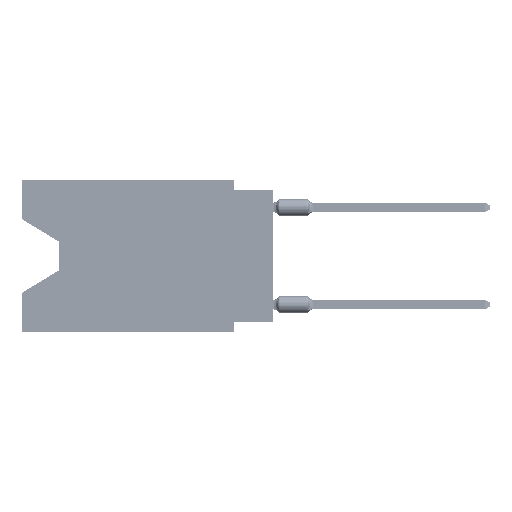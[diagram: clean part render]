
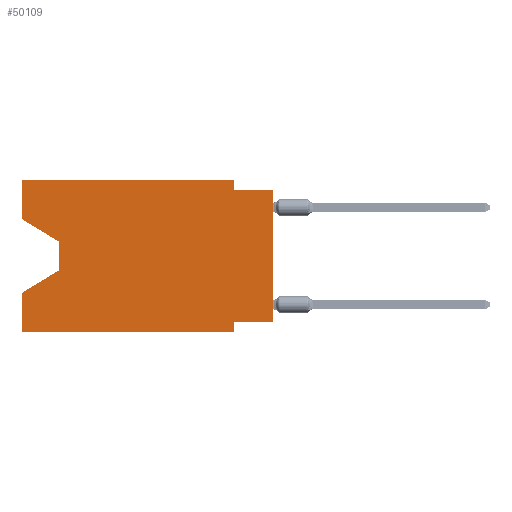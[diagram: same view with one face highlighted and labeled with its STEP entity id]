
A CAD part, left-side view. The second image highlights one B-rep face of the part: STEP entity #50109.
In plain terms, the highlighted planar face has unit normal (-1, 0, 0).
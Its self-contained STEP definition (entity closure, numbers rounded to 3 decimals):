
#294 = VECTOR ( 'NONE', #69020, 1000. ) ;
#540 = DIRECTION ( 'NONE',  ( 0., -0.855, -0.519 ) ) ;
#623 = VECTOR ( 'NONE', #20585, 1000. ) ;
#2536 = VECTOR ( 'NONE', #59186, 1000. ) ;
#3504 = LINE ( 'NONE', #13956, #27355 ) ;
#3783 = LINE ( 'NONE', #47418, #16172 ) ;
#3912 = CARTESIAN_POINT ( 'NONE',  ( 0., 0., -0.635 ) ) ;
#4102 = CARTESIAN_POINT ( 'NONE',  ( 0., 2.54, -0.635 ) ) ;
#5172 = EDGE_CURVE ( 'NONE', #53596, #12329, #67324, .T. ) ;
#5180 = DIRECTION ( 'NONE',  ( 0., 0., -1. ) ) ;
#5236 = CARTESIAN_POINT ( 'NONE',  ( 0., 2.54, 0. ) ) ;
#5905 = ORIENTED_EDGE ( 'NONE', *, *, #60990, .F. ) ;
#6572 = EDGE_CURVE ( 'NONE', #6758, #55986, #24135, .T. ) ;
#6710 = EDGE_CURVE ( 'NONE', #51719, #12329, #8767, .T. ) ;
#6758 = VERTEX_POINT ( 'NONE', #38417 ) ;
#7532 = VERTEX_POINT ( 'NONE', #47621 ) ;
#7978 = CARTESIAN_POINT ( 'NONE',  ( 0., 13.97, -5.893 ) ) ;
#8767 = LINE ( 'NONE', #68135, #49647 ) ;
#10934 = EDGE_CURVE ( 'NONE', #21162, #53596, #31656, .T. ) ;
#11527 = DIRECTION ( 'NONE',  ( 0., 0., -1. ) ) ;
#12329 = VERTEX_POINT ( 'NONE', #28483 ) ;
#13956 = CARTESIAN_POINT ( 'NONE',  ( 0., 16.383, 0. ) ) ;
#16172 = VECTOR ( 'NONE', #20525, 1000. ) ;
#16595 = CARTESIAN_POINT ( 'NONE',  ( 0., 16.383, -2.546 ) ) ;
#17755 = VERTEX_POINT ( 'NONE', #43179 ) ;
#20525 = DIRECTION ( 'NONE',  ( 0., 0., 1. ) ) ;
#20585 = DIRECTION ( 'NONE',  ( 0., 0.855, -0.519 ) ) ;
#21162 = VERTEX_POINT ( 'NONE', #23049 ) ;
#21661 = CARTESIAN_POINT ( 'NONE',  ( 0., 2.54, 0. ) ) ;
#22603 = CARTESIAN_POINT ( 'NONE',  ( 0., 16.383, 0. ) ) ;
#23049 = CARTESIAN_POINT ( 'NONE',  ( 0., 0., -9.271 ) ) ;
#24135 = LINE ( 'NONE', #61195, #56314 ) ;
#25287 = VECTOR ( 'NONE', #30642, 1000. ) ;
#25675 = ORIENTED_EDGE ( 'NONE', *, *, #6710, .T. ) ;
#25848 = ORIENTED_EDGE ( 'NONE', *, *, #32388, .F. ) ;
#27098 = LINE ( 'NONE', #16595, #43130 ) ;
#27355 = VECTOR ( 'NONE', #46805, 1000. ) ;
#27444 = DIRECTION ( 'NONE',  ( 0., 1., 0. ) ) ;
#27961 = ORIENTED_EDGE ( 'NONE', *, *, #65818, .F. ) ;
#28483 = CARTESIAN_POINT ( 'NONE',  ( 0., 2.54, -9.906 ) ) ;
#29732 = DIRECTION ( 'NONE',  ( 0., -1., 0. ) ) ;
#29880 = AXIS2_PLACEMENT_3D ( 'NONE', #41851, #31728, #5180 ) ;
#30098 = DIRECTION ( 'NONE',  ( 0., -1., 0. ) ) ;
#30329 = ORIENTED_EDGE ( 'NONE', *, *, #45778, .F. ) ;
#30642 = DIRECTION ( 'NONE',  ( 0., 0., -1. ) ) ;
#30957 = LINE ( 'NONE', #48055, #294 ) ;
#31656 = LINE ( 'NONE', #52958, #46522 ) ;
#31728 = DIRECTION ( 'NONE',  ( 1., 0., 0. ) ) ;
#31939 = LINE ( 'NONE', #58147, #2536 ) ;
#32388 = EDGE_CURVE ( 'NONE', #54689, #66324, #38411, .T. ) ;
#34067 = VERTEX_POINT ( 'NONE', #3912 ) ;
#38411 = LINE ( 'NONE', #21661, #49510 ) ;
#38417 = CARTESIAN_POINT ( 'NONE',  ( 0., 13.97, -4.013 ) ) ;
#39183 = DIRECTION ( 'NONE',  ( 0., 0., -1. ) ) ;
#41786 = ORIENTED_EDGE ( 'NONE', *, *, #48623, .T. ) ;
#41851 = CARTESIAN_POINT ( 'NONE',  ( 0., 16.383, 0. ) ) ;
#42254 = CARTESIAN_POINT ( 'NONE',  ( 0., 2.54, -9.271 ) ) ;
#42256 = LINE ( 'NONE', #59036, #623 ) ;
#42548 = FACE_OUTER_BOUND ( 'NONE', #49170, .T. ) ;
#43130 = VECTOR ( 'NONE', #540, 1000. ) ;
#43179 = CARTESIAN_POINT ( 'NONE',  ( 0., 16.383, -7.36 ) ) ;
#43508 = ORIENTED_EDGE ( 'NONE', *, *, #10934, .F. ) ;
#44022 = ORIENTED_EDGE ( 'NONE', *, *, #6572, .T. ) ;
#45778 = EDGE_CURVE ( 'NONE', #65018, #54689, #46466, .T. ) ;
#46466 = LINE ( 'NONE', #47170, #50040 ) ;
#46522 = VECTOR ( 'NONE', #27444, 1000. ) ;
#46805 = DIRECTION ( 'NONE',  ( 0., 0., 1. ) ) ;
#46900 = EDGE_CURVE ( 'NONE', #7532, #65018, #3783, .T. ) ;
#47170 = CARTESIAN_POINT ( 'NONE',  ( 0., 16.383, 0. ) ) ;
#47418 = CARTESIAN_POINT ( 'NONE',  ( 0., 16.383, 0. ) ) ;
#47621 = CARTESIAN_POINT ( 'NONE',  ( 0., 16.383, -2.546 ) ) ;
#48055 = CARTESIAN_POINT ( 'NONE',  ( 0., 0., 0. ) ) ;
#48623 = EDGE_CURVE ( 'NONE', #7532, #6758, #27098, .T. ) ;
#49170 = EDGE_LOOP ( 'NONE', ( #41786, #44022, #50064, #27961, #25675, #57112, #43508, #57638, #5905, #25848, #30329, #62184 ) ) ;
#49510 = VECTOR ( 'NONE', #11527, 1000. ) ;
#49647 = VECTOR ( 'NONE', #30098, 1000. ) ;
#50040 = VECTOR ( 'NONE', #29732, 1000. ) ;
#50064 = ORIENTED_EDGE ( 'NONE', *, *, #66075, .T. ) ;
#50109 = ADVANCED_FACE ( 'NONE', ( #42548 ), #57940, .F. ) ;
#51719 = VERTEX_POINT ( 'NONE', #51935 ) ;
#51935 = CARTESIAN_POINT ( 'NONE',  ( 0., 16.383, -9.906 ) ) ;
#51950 = CARTESIAN_POINT ( 'NONE',  ( 0., 2.54, -9.906 ) ) ;
#52958 = CARTESIAN_POINT ( 'NONE',  ( 0., 0., -9.271 ) ) ;
#53596 = VERTEX_POINT ( 'NONE', #42254 ) ;
#54689 = VERTEX_POINT ( 'NONE', #5236 ) ;
#55986 = VERTEX_POINT ( 'NONE', #7978 ) ;
#56314 = VECTOR ( 'NONE', #39183, 1000. ) ;
#57112 = ORIENTED_EDGE ( 'NONE', *, *, #5172, .F. ) ;
#57638 = ORIENTED_EDGE ( 'NONE', *, *, #62612, .T. ) ;
#57940 = PLANE ( 'NONE',  #29880 ) ;
#58147 = CARTESIAN_POINT ( 'NONE',  ( 0., 0., -0.635 ) ) ;
#59036 = CARTESIAN_POINT ( 'NONE',  ( 0., 13.97, -5.893 ) ) ;
#59186 = DIRECTION ( 'NONE',  ( 0., -1., 0. ) ) ;
#60990 = EDGE_CURVE ( 'NONE', #66324, #34067, #31939, .T. ) ;
#61195 = CARTESIAN_POINT ( 'NONE',  ( 0., 13.97, -4.013 ) ) ;
#62184 = ORIENTED_EDGE ( 'NONE', *, *, #46900, .F. ) ;
#62612 = EDGE_CURVE ( 'NONE', #21162, #34067, #30957, .T. ) ;
#65018 = VERTEX_POINT ( 'NONE', #22603 ) ;
#65818 = EDGE_CURVE ( 'NONE', #51719, #17755, #3504, .T. ) ;
#66075 = EDGE_CURVE ( 'NONE', #55986, #17755, #42256, .T. ) ;
#66324 = VERTEX_POINT ( 'NONE', #4102 ) ;
#67324 = LINE ( 'NONE', #51950, #25287 ) ;
#68135 = CARTESIAN_POINT ( 'NONE',  ( 0., 16.383, -9.906 ) ) ;
#69020 = DIRECTION ( 'NONE',  ( 0., 0., 1. ) ) ;
